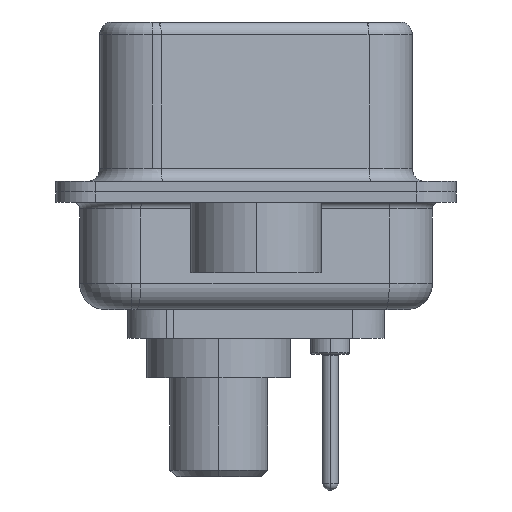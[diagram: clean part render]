
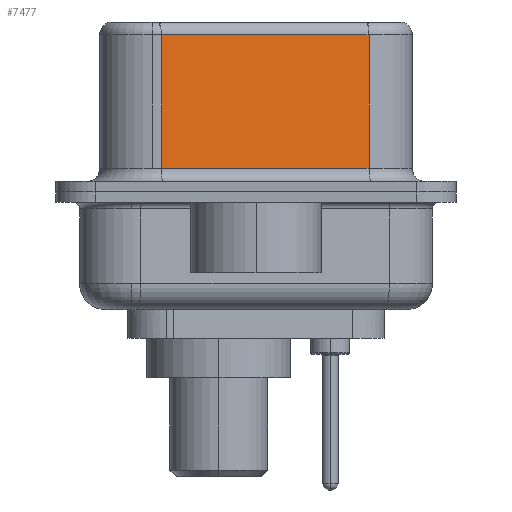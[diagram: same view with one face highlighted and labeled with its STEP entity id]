
A CAD part, left-side view. The second image highlights one B-rep face of the part: STEP entity #7477.
In plain terms, the highlighted planar face has unit normal (-0.985, -0.174, 0).
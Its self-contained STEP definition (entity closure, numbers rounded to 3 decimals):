
#567 = CARTESIAN_POINT ( 'NONE',  ( 5.132, -4.322, 6.52 ) ) ;
#1158 = LINE ( 'NONE', #16625, #13594 ) ;
#3139 = CARTESIAN_POINT ( 'NONE',  ( 5.132, -4.322, 6.52 ) ) ;
#3576 = DIRECTION ( 'NONE',  ( 0., 0., -1. ) ) ;
#4171 = VECTOR ( 'NONE', #9658, 1000. ) ;
#4423 = ORIENTED_EDGE ( 'NONE', *, *, #5169, .T. ) ;
#4754 = AXIS2_PLACEMENT_3D ( 'NONE', #3139, #18875, #19974 ) ;
#5169 = EDGE_CURVE ( 'NONE', #7738, #12562, #12766, .T. ) ;
#5249 = EDGE_CURVE ( 'NONE', #16589, #18143, #20008, .T. ) ;
#6317 = CARTESIAN_POINT ( 'NONE',  ( 5.132, -4.322, 0.9 ) ) ;
#6618 = ORIENTED_EDGE ( 'NONE', *, *, #12171, .T. ) ;
#7438 = CARTESIAN_POINT ( 'NONE',  ( 5.132, -4.322, 6.02 ) ) ;
#7477 = ADVANCED_FACE ( 'NONE', ( #14392 ), #15357, .F. ) ;
#7738 = VERTEX_POINT ( 'NONE', #17629 ) ;
#7795 = ORIENTED_EDGE ( 'NONE', *, *, #20388, .T. ) ;
#9658 = DIRECTION ( 'NONE',  ( 0., 0., -1. ) ) ;
#11229 = VECTOR ( 'NONE', #3576, 1000. ) ;
#11695 = DIRECTION ( 'NONE',  ( 0.174, -0.985, 0. ) ) ;
#12171 = EDGE_CURVE ( 'NONE', #16589, #7738, #13723, .T. ) ;
#12562 = VERTEX_POINT ( 'NONE', #20034 ) ;
#12766 = LINE ( 'NONE', #19159, #4171 ) ;
#12981 = EDGE_LOOP ( 'NONE', ( #14733, #6618, #4423, #7795 ) ) ;
#13204 = VECTOR ( 'NONE', #17138, 1000. ) ;
#13594 = VECTOR ( 'NONE', #11695, 1000. ) ;
#13723 = LINE ( 'NONE', #7438, #13204 ) ;
#14010 = CARTESIAN_POINT ( 'NONE',  ( 5.132, -4.322, 6.02 ) ) ;
#14392 = FACE_OUTER_BOUND ( 'NONE', #12981, .T. ) ;
#14733 = ORIENTED_EDGE ( 'NONE', *, *, #5249, .F. ) ;
#15357 = PLANE ( 'NONE',  #4754 ) ;
#16589 = VERTEX_POINT ( 'NONE', #14010 ) ;
#16625 = CARTESIAN_POINT ( 'NONE',  ( 5.132, -4.322, 0.9 ) ) ;
#17138 = DIRECTION ( 'NONE',  ( -0.174, 0.985, 0. ) ) ;
#17629 = CARTESIAN_POINT ( 'NONE',  ( 3.73, 3.628, 6.02 ) ) ;
#18143 = VERTEX_POINT ( 'NONE', #6317 ) ;
#18875 = DIRECTION ( 'NONE',  ( 0.985, 0.174, 0. ) ) ;
#19159 = CARTESIAN_POINT ( 'NONE',  ( 3.73, 3.628, 6.52 ) ) ;
#19974 = DIRECTION ( 'NONE',  ( -0.174, 0.985, 0. ) ) ;
#20008 = LINE ( 'NONE', #567, #11229 ) ;
#20034 = CARTESIAN_POINT ( 'NONE',  ( 3.73, 3.628, 0.9 ) ) ;
#20388 = EDGE_CURVE ( 'NONE', #12562, #18143, #1158, .T. ) ;
